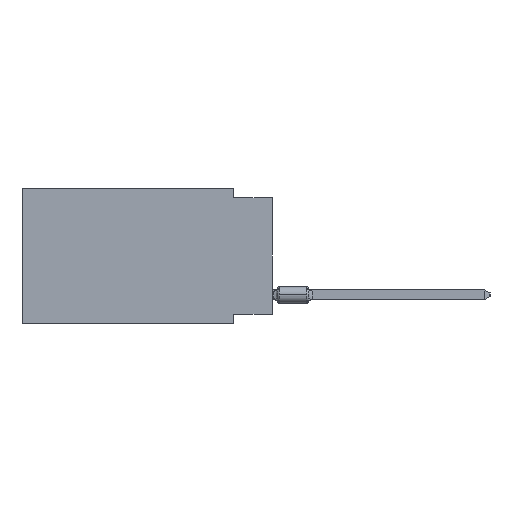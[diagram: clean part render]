
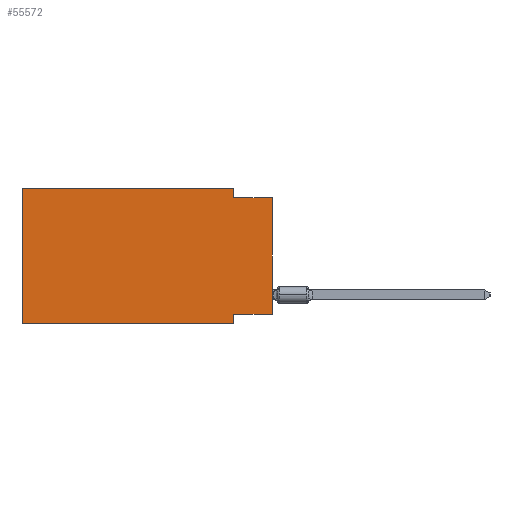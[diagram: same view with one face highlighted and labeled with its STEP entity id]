
A CAD part, left-side view. The second image highlights one B-rep face of the part: STEP entity #55572.
In plain terms, the highlighted planar face has unit normal (-1, 0, 0).
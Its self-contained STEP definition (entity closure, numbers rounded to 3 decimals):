
#2547 = EDGE_CURVE ( 'NONE', #38406, #37148, #5467, .T. ) ;
#3754 = ORIENTED_EDGE ( 'NONE', *, *, #59252, .F. ) ;
#4764 = DIRECTION ( 'NONE',  ( 0., 0., 1. ) ) ;
#5467 = LINE ( 'NONE', #26228, #15098 ) ;
#8020 = VECTOR ( 'NONE', #8135, 1000. ) ;
#8135 = DIRECTION ( 'NONE',  ( 0., -1., 0. ) ) ;
#9440 = CARTESIAN_POINT ( 'NONE',  ( 0., 0., 0. ) ) ;
#9622 = VERTEX_POINT ( 'NONE', #30337 ) ;
#12045 = DIRECTION ( 'NONE',  ( 0., 0., -1. ) ) ;
#14258 = CARTESIAN_POINT ( 'NONE',  ( 0., 16.383, 0. ) ) ;
#14415 = DIRECTION ( 'NONE',  ( 0., 0., -1. ) ) ;
#15098 = VECTOR ( 'NONE', #4764, 1000. ) ;
#15300 = VERTEX_POINT ( 'NONE', #30404 ) ;
#16954 = LINE ( 'NONE', #66276, #65870 ) ;
#18179 = VERTEX_POINT ( 'NONE', #26392 ) ;
#21319 = VECTOR ( 'NONE', #69396, 1000. ) ;
#23640 = ORIENTED_EDGE ( 'NONE', *, *, #60733, .F. ) ;
#25156 = LINE ( 'NONE', #63374, #25185 ) ;
#25185 = VECTOR ( 'NONE', #14415, 1000. ) ;
#25271 = PLANE ( 'NONE',  #49509 ) ;
#26228 = CARTESIAN_POINT ( 'NONE',  ( 0., 16.383, 0. ) ) ;
#26392 = CARTESIAN_POINT ( 'NONE',  ( 0., 2.54, -8.89 ) ) ;
#27500 = ORIENTED_EDGE ( 'NONE', *, *, #2547, .F. ) ;
#27702 = DIRECTION ( 'NONE',  ( 0., -1., 0. ) ) ;
#28473 = ORIENTED_EDGE ( 'NONE', *, *, #31606, .T. ) ;
#30337 = CARTESIAN_POINT ( 'NONE',  ( 0., 2.54, 0. ) ) ;
#30404 = CARTESIAN_POINT ( 'NONE',  ( 0., 0., -0.635 ) ) ;
#31346 = DIRECTION ( 'NONE',  ( 0., 0., -1. ) ) ;
#31606 = EDGE_CURVE ( 'NONE', #38406, #18179, #16954, .T. ) ;
#36197 = EDGE_LOOP ( 'NONE', ( #59229, #58154, #23640, #56657, #27500, #28473, #57615, #3754 ) ) ;
#37057 = CARTESIAN_POINT ( 'NONE',  ( 0., 16.383, 0. ) ) ;
#37148 = VERTEX_POINT ( 'NONE', #14258 ) ;
#38406 = VERTEX_POINT ( 'NONE', #51235 ) ;
#42294 = VECTOR ( 'NONE', #63164, 1000. ) ;
#43119 = DIRECTION ( 'NONE',  ( 1., 0., 0. ) ) ;
#47858 = VECTOR ( 'NONE', #57699, 1000. ) ;
#48822 = CARTESIAN_POINT ( 'NONE',  ( 0., 2.54, -8.255 ) ) ;
#49444 = EDGE_CURVE ( 'NONE', #37148, #9622, #57097, .T. ) ;
#49509 = AXIS2_PLACEMENT_3D ( 'NONE', #37057, #43119, #31346 ) ;
#49677 = EDGE_CURVE ( 'NONE', #53134, #15300, #63858, .T. ) ;
#50133 = EDGE_CURVE ( 'NONE', #57259, #15300, #52697, .T. ) ;
#51235 = CARTESIAN_POINT ( 'NONE',  ( 0., 16.383, -8.89 ) ) ;
#51403 = CARTESIAN_POINT ( 'NONE',  ( 0., 16.383, 0. ) ) ;
#52697 = LINE ( 'NONE', #9440, #47858 ) ;
#53134 = VERTEX_POINT ( 'NONE', #70650 ) ;
#54012 = CARTESIAN_POINT ( 'NONE',  ( 0., 0., -8.255 ) ) ;
#55572 = ADVANCED_FACE ( 'NONE', ( #63849 ), #25271, .F. ) ;
#55647 = LINE ( 'NONE', #61006, #68733 ) ;
#56657 = ORIENTED_EDGE ( 'NONE', *, *, #49444, .F. ) ;
#57097 = LINE ( 'NONE', #51403, #8020 ) ;
#57259 = VERTEX_POINT ( 'NONE', #63419 ) ;
#57615 = ORIENTED_EDGE ( 'NONE', *, *, #66899, .F. ) ;
#57699 = DIRECTION ( 'NONE',  ( 0., 0., 1. ) ) ;
#58154 = ORIENTED_EDGE ( 'NONE', *, *, #49677, .F. ) ;
#58648 = LINE ( 'NONE', #54012, #21319 ) ;
#59229 = ORIENTED_EDGE ( 'NONE', *, *, #50133, .T. ) ;
#59252 = EDGE_CURVE ( 'NONE', #57259, #59861, #58648, .T. ) ;
#59861 = VERTEX_POINT ( 'NONE', #48822 ) ;
#60733 = EDGE_CURVE ( 'NONE', #9622, #53134, #55647, .T. ) ;
#61006 = CARTESIAN_POINT ( 'NONE',  ( 0., 2.54, 0. ) ) ;
#63164 = DIRECTION ( 'NONE',  ( 0., -1., 0. ) ) ;
#63374 = CARTESIAN_POINT ( 'NONE',  ( 0., 2.54, -8.89 ) ) ;
#63419 = CARTESIAN_POINT ( 'NONE',  ( 0., 0., -8.255 ) ) ;
#63849 = FACE_OUTER_BOUND ( 'NONE', #36197, .T. ) ;
#63858 = LINE ( 'NONE', #64208, #42294 ) ;
#64208 = CARTESIAN_POINT ( 'NONE',  ( 0., 0., -0.635 ) ) ;
#65870 = VECTOR ( 'NONE', #27702, 1000. ) ;
#66276 = CARTESIAN_POINT ( 'NONE',  ( 0., 16.383, -8.89 ) ) ;
#66899 = EDGE_CURVE ( 'NONE', #59861, #18179, #25156, .T. ) ;
#68733 = VECTOR ( 'NONE', #12045, 1000. ) ;
#69396 = DIRECTION ( 'NONE',  ( 0., 1., 0. ) ) ;
#70650 = CARTESIAN_POINT ( 'NONE',  ( 0., 2.54, -0.635 ) ) ;
